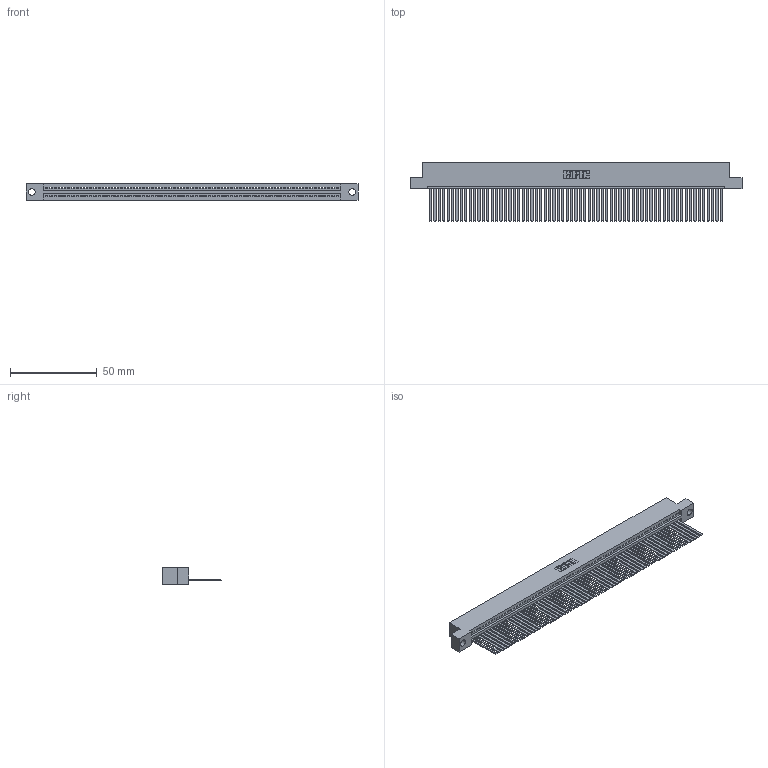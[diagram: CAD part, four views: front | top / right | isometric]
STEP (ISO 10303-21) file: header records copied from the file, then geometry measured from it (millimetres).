
FILE_DESCRIPTION (( 'STEP AP203' ), '1' );
FILE_NAME ('395-067-544-104.STEP', '2018-11-25T10:35:15', ( '' ), ( '' ), 'SwSTEP 2.0', 'SolidWorks 2016', '' );
FILE_SCHEMA (( 'CONFIG_CONTROL_DESIGN' ));
Length unit declared in the file: inch
Products named in the file (3): 345 Part_Flush Mounting Lugs - 0.156 Dia-TH; 395-067-544-104; 345-292-001_345-293-144
Assembly tree (68 placements, depth 2):
  395-067-544-104
    345 Part_Flush Mounting Lugs - 0.156 Dia-TH
    345-292-001_345-293-144  x67
Bounding box: 191.39 x 33.96 x 9.4 mm (x, y, z)
Volume: 19071.2 mm3; surface area: 27821.9 mm2
Topology: 68 solids, 68 shells, 3610 faces, 10927 edges, 7194 vertices
Faces by surface type: plane 2492, cylinder 1118
Entity records: 46879 total; most frequent: ORIENTED_EDGE 8126, CARTESIAN_POINT 8125, DIRECTION 7057, EDGE_CURVE 4063, VECTOR 3667, LINE 3667, VERTEX_POINT 2706, AXIS2_PLACEMENT_3D 1695
